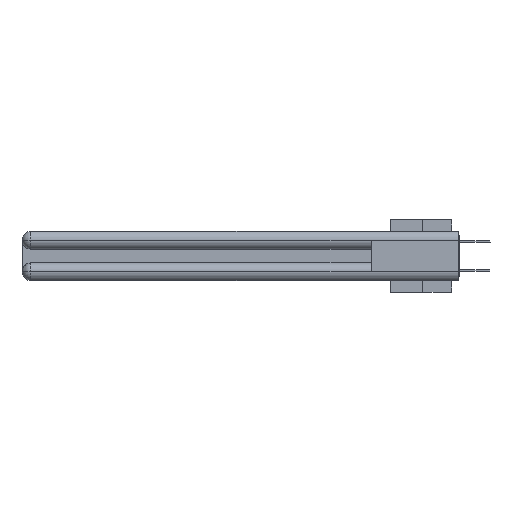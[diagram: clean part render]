
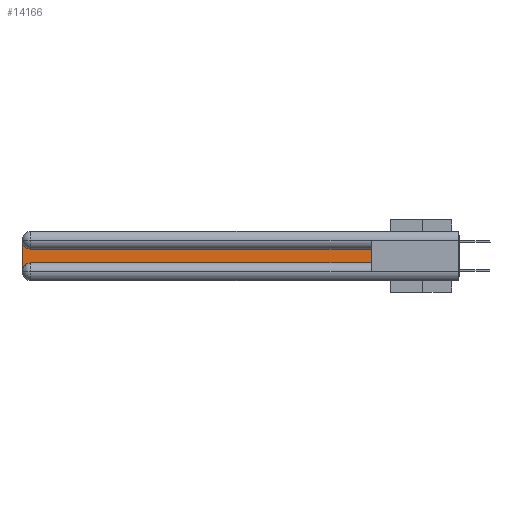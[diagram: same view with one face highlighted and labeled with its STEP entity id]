
A CAD part, left-side view. The second image highlights one B-rep face of the part: STEP entity #14166.
In plain terms, the highlighted planar face has unit normal (-1, 0, 0).
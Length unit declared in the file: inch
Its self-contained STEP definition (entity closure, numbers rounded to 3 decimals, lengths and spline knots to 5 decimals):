
#631 = CIRCLE ( 'NONE', #27379, 0.06 ) ;
#1033 = AXIS2_PLACEMENT_3D ( 'NONE', #12378, #17744, #25287 ) ;
#1417 = DIRECTION ( 'NONE',  ( 0., 0., 1. ) ) ;
#4475 = ORIENTED_EDGE ( 'NONE', *, *, #20509, .T. ) ;
#5815 = CARTESIAN_POINT ( 'NONE',  ( 0.075, 0.6, -0.1225 ) ) ;
#6612 = DIRECTION ( 'NONE',  ( 0., 1., 0. ) ) ;
#6672 = DIRECTION ( 'NONE',  ( 0., -1., 0. ) ) ;
#7347 = VERTEX_POINT ( 'NONE', #5815 ) ;
#7901 = CIRCLE ( 'NONE', #30354, 0.06 ) ;
#8101 = VERTEX_POINT ( 'NONE', #10554 ) ;
#8492 = DIRECTION ( 'NONE',  ( 0., 0., -1. ) ) ;
#8635 = VECTOR ( 'NONE', #6612, 39.37008 ) ;
#10554 = CARTESIAN_POINT ( 'NONE',  ( 0.075, 2.94, -0.2175 ) ) ;
#11766 = VERTEX_POINT ( 'NONE', #18888 ) ;
#12171 = CARTESIAN_POINT ( 'NONE',  ( 0.075, 0.6, -0.2175 ) ) ;
#12378 = CARTESIAN_POINT ( 'NONE',  ( 0.075, 3., -0.1225 ) ) ;
#12390 = DIRECTION ( 'NONE',  ( 0., 0., -1. ) ) ;
#12567 = LINE ( 'NONE', #27978, #29050 ) ;
#13147 = VERTEX_POINT ( 'NONE', #18593 ) ;
#14133 = CARTESIAN_POINT ( 'NONE',  ( 0.075, 0.6, -0.1225 ) ) ;
#14166 = ADVANCED_FACE ( 'NONE', ( #19932 ), #27296, .F. ) ;
#15304 = VERTEX_POINT ( 'NONE', #18153 ) ;
#15659 = CARTESIAN_POINT ( 'NONE',  ( 0.075, 3., -0.0625 ) ) ;
#16142 = ORIENTED_EDGE ( 'NONE', *, *, #23686, .T. ) ;
#16302 = EDGE_CURVE ( 'NONE', #11766, #18081, #7901, .T. ) ;
#16773 = DIRECTION ( 'NONE',  ( 0., 0., -1. ) ) ;
#17376 = LINE ( 'NONE', #12171, #29408 ) ;
#17744 = DIRECTION ( 'NONE',  ( 1., 0., 0. ) ) ;
#18081 = VERTEX_POINT ( 'NONE', #15659 ) ;
#18153 = CARTESIAN_POINT ( 'NONE',  ( 0.075, 3., -0.2775 ) ) ;
#18593 = CARTESIAN_POINT ( 'NONE',  ( 0.075, 0.6, -0.2175 ) ) ;
#18874 = VECTOR ( 'NONE', #1417, 39.37008 ) ;
#18888 = CARTESIAN_POINT ( 'NONE',  ( 0.075, 2.94, -0.1225 ) ) ;
#19490 = LINE ( 'NONE', #14133, #8635 ) ;
#19847 = LINE ( 'NONE', #22528, #18874 ) ;
#19932 = FACE_OUTER_BOUND ( 'NONE', #25073, .T. ) ;
#20509 = EDGE_CURVE ( 'NONE', #8101, #13147, #17376, .T. ) ;
#21205 = CARTESIAN_POINT ( 'NONE',  ( 0.075, 2.94, -0.0625 ) ) ;
#22528 = CARTESIAN_POINT ( 'NONE',  ( 0.075, 0.6, -0.2175 ) ) ;
#23203 = ORIENTED_EDGE ( 'NONE', *, *, #29806, .T. ) ;
#23686 = EDGE_CURVE ( 'NONE', #13147, #7347, #19847, .T. ) ;
#23967 = CARTESIAN_POINT ( 'NONE',  ( 0.075, 2.94, -0.2775 ) ) ;
#24130 = DIRECTION ( 'NONE',  ( 1., 0., 0. ) ) ;
#25073 = EDGE_LOOP ( 'NONE', ( #23203, #31678, #31033, #30207, #4475, #16142 ) ) ;
#25287 = DIRECTION ( 'NONE',  ( 0., 0., -1. ) ) ;
#26001 = EDGE_CURVE ( 'NONE', #18081, #15304, #12567, .T. ) ;
#27296 = PLANE ( 'NONE',  #1033 ) ;
#27379 = AXIS2_PLACEMENT_3D ( 'NONE', #23967, #24130, #16773 ) ;
#27978 = CARTESIAN_POINT ( 'NONE',  ( 0.075, 3., -0.2175 ) ) ;
#29050 = VECTOR ( 'NONE', #12390, 39.37008 ) ;
#29408 = VECTOR ( 'NONE', #6672, 39.37008 ) ;
#29806 = EDGE_CURVE ( 'NONE', #7347, #11766, #19490, .T. ) ;
#30207 = ORIENTED_EDGE ( 'NONE', *, *, #30342, .T. ) ;
#30342 = EDGE_CURVE ( 'NONE', #15304, #8101, #631, .T. ) ;
#30354 = AXIS2_PLACEMENT_3D ( 'NONE', #21205, #31402, #8492 ) ;
#31033 = ORIENTED_EDGE ( 'NONE', *, *, #26001, .T. ) ;
#31402 = DIRECTION ( 'NONE',  ( 1., 0., 0. ) ) ;
#31678 = ORIENTED_EDGE ( 'NONE', *, *, #16302, .T. ) ;
